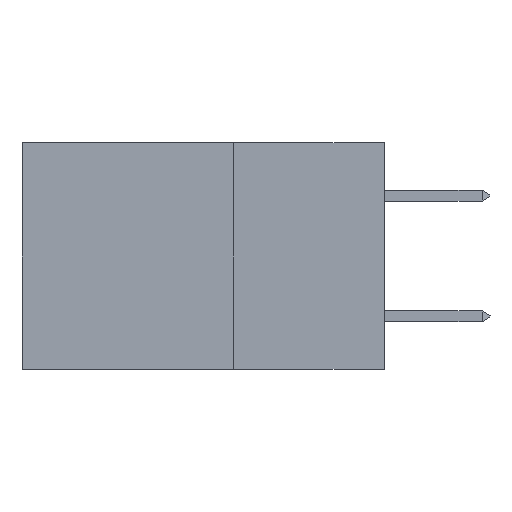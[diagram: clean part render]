
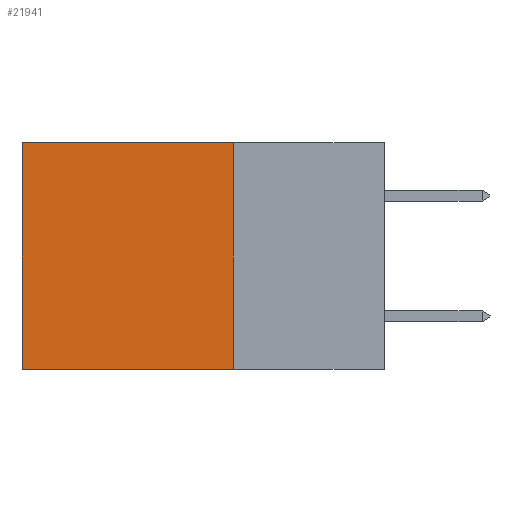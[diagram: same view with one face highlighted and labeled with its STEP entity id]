
A CAD part, left-side view. The second image highlights one B-rep face of the part: STEP entity #21941.
In plain terms, the highlighted planar face has unit normal (-1, 0, 0).
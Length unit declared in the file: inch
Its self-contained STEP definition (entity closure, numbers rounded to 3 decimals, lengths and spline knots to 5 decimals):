
#1067 = EDGE_LOOP ( 'NONE', ( #12857, #20286, #15414, #6063 ) ) ;
#1734 = VERTEX_POINT ( 'NONE', #9515 ) ;
#3245 = DIRECTION ( 'NONE',  ( 0., 1., 0. ) ) ;
#4317 = LINE ( 'NONE', #20170, #7104 ) ;
#4543 = LINE ( 'NONE', #15106, #8159 ) ;
#6063 = ORIENTED_EDGE ( 'NONE', *, *, #22829, .T. ) ;
#6385 = CARTESIAN_POINT ( 'NONE',  ( 0.2875, 0.6, -0.375 ) ) ;
#7104 = VECTOR ( 'NONE', #9521, 39.37008 ) ;
#7899 = VECTOR ( 'NONE', #3245, 39.37008 ) ;
#8056 = PLANE ( 'NONE',  #16378 ) ;
#8159 = VECTOR ( 'NONE', #16903, 39.37008 ) ;
#8210 = DIRECTION ( 'NONE',  ( 0., 0., -1. ) ) ;
#9128 = VERTEX_POINT ( 'NONE', #9656 ) ;
#9515 = CARTESIAN_POINT ( 'NONE',  ( 0.2875, 0.6, -0.375 ) ) ;
#9521 = DIRECTION ( 'NONE',  ( 0., 0., -1. ) ) ;
#9656 = CARTESIAN_POINT ( 'NONE',  ( 0.2875, 0.25, -0.375 ) ) ;
#11743 = EDGE_CURVE ( 'NONE', #9128, #1734, #12130, .T. ) ;
#11763 = CARTESIAN_POINT ( 'NONE',  ( 0.2875, 0.25, -0.375 ) ) ;
#12130 = LINE ( 'NONE', #16060, #7899 ) ;
#12857 = ORIENTED_EDGE ( 'NONE', *, *, #19377, .T. ) ;
#13338 = CARTESIAN_POINT ( 'NONE',  ( 0.2875, 0.6, 0. ) ) ;
#13543 = VERTEX_POINT ( 'NONE', #13338 ) ;
#14737 = VERTEX_POINT ( 'NONE', #20977 ) ;
#15106 = CARTESIAN_POINT ( 'NONE',  ( 0.2875, 0.25, 0. ) ) ;
#15414 = ORIENTED_EDGE ( 'NONE', *, *, #17029, .F. ) ;
#16060 = CARTESIAN_POINT ( 'NONE',  ( 0.2875, 0.25, -0.375 ) ) ;
#16181 = VECTOR ( 'NONE', #20625, 39.37008 ) ;
#16378 = AXIS2_PLACEMENT_3D ( 'NONE', #11763, #18781, #8210 ) ;
#16903 = DIRECTION ( 'NONE',  ( 0., 1., 0. ) ) ;
#17029 = EDGE_CURVE ( 'NONE', #14737, #9128, #4317, .T. ) ;
#17789 = FACE_OUTER_BOUND ( 'NONE', #1067, .T. ) ;
#18781 = DIRECTION ( 'NONE',  ( 1., 0., 0. ) ) ;
#19377 = EDGE_CURVE ( 'NONE', #13543, #1734, #22101, .T. ) ;
#20170 = CARTESIAN_POINT ( 'NONE',  ( 0.2875, 0.25, -0.375 ) ) ;
#20286 = ORIENTED_EDGE ( 'NONE', *, *, #11743, .F. ) ;
#20625 = DIRECTION ( 'NONE',  ( 0., 0., -1. ) ) ;
#20977 = CARTESIAN_POINT ( 'NONE',  ( 0.2875, 0.25, 0. ) ) ;
#21941 = ADVANCED_FACE ( 'NONE', ( #17789 ), #8056, .F. ) ;
#22101 = LINE ( 'NONE', #6385, #16181 ) ;
#22829 = EDGE_CURVE ( 'NONE', #14737, #13543, #4543, .T. ) ;
